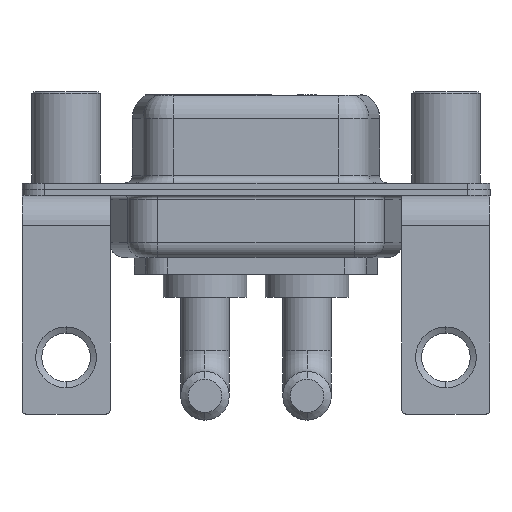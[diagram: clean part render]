
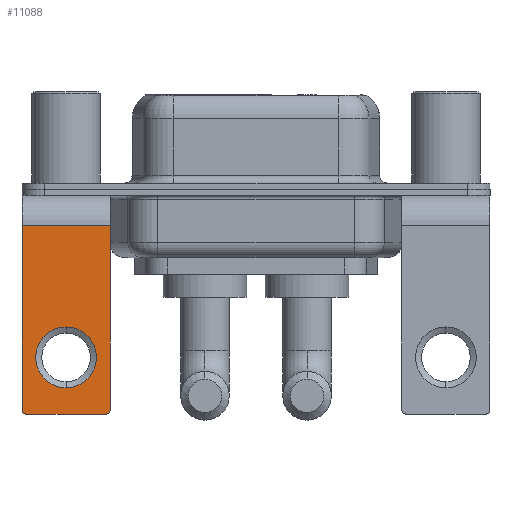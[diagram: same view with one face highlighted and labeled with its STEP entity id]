
A CAD part, front view. The second image highlights one B-rep face of the part: STEP entity #11088.
In plain terms, the highlighted planar face has unit normal (0, -1, 0).
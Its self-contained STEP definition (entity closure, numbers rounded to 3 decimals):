
#146 = LINE ( 'NONE', #1352, #6501 ) ;
#164 = ORIENTED_EDGE ( 'NONE', *, *, #9852, .F. ) ;
#209 = VECTOR ( 'NONE', #15672, 1000. ) ;
#387 = AXIS2_PLACEMENT_3D ( 'NONE', #13429, #12465, #3819 ) ;
#992 = VERTEX_POINT ( 'NONE', #1568 ) ;
#1039 = VERTEX_POINT ( 'NONE', #6690 ) ;
#1127 = VERTEX_POINT ( 'NONE', #11657 ) ;
#1352 = CARTESIAN_POINT ( 'NONE',  ( 2.9, -6.25, -14.8 ) ) ;
#1568 = CARTESIAN_POINT ( 'NONE',  ( 2.65, -6.25, -14.8 ) ) ;
#1747 = ORIENTED_EDGE ( 'NONE', *, *, #2289, .T. ) ;
#1815 = CIRCLE ( 'NONE', #6667, 0.25 ) ;
#2026 = CARTESIAN_POINT ( 'NONE',  ( 2.65, -6.25, -14.55 ) ) ;
#2289 = EDGE_CURVE ( 'NONE', #1127, #10317, #7300, .T. ) ;
#2880 = EDGE_CURVE ( 'NONE', #12796, #14570, #13454, .T. ) ;
#3440 = CIRCLE ( 'NONE', #14408, 0.25 ) ;
#3556 = VECTOR ( 'NONE', #14401, 1000. ) ;
#3585 = EDGE_LOOP ( 'NONE', ( #1747, #15638 ) ) ;
#3605 = CARTESIAN_POINT ( 'NONE',  ( 2.9, -6.25, -2.4 ) ) ;
#3757 = DIRECTION ( 'NONE',  ( 0., 0., 1. ) ) ;
#3819 = DIRECTION ( 'NONE',  ( 0., 0., 1. ) ) ;
#4032 = LINE ( 'NONE', #4910, #9857 ) ;
#4249 = DIRECTION ( 'NONE',  ( 0., 0., 1. ) ) ;
#4501 = CARTESIAN_POINT ( 'NONE',  ( 2.9, -6.25, -2.4 ) ) ;
#4638 = ORIENTED_EDGE ( 'NONE', *, *, #9647, .T. ) ;
#4791 = ORIENTED_EDGE ( 'NONE', *, *, #12128, .T. ) ;
#4910 = CARTESIAN_POINT ( 'NONE',  ( -2.9, -6.25, -2.4 ) ) ;
#4927 = EDGE_CURVE ( 'NONE', #10317, #1127, #7939, .T. ) ;
#4948 = EDGE_CURVE ( 'NONE', #992, #9258, #1815, .T. ) ;
#5245 = EDGE_LOOP ( 'NONE', ( #4791, #4638, #164, #15723, #7160, #8652 ) ) ;
#5376 = CARTESIAN_POINT ( 'NONE',  ( 0., -6.25, -11.07 ) ) ;
#6077 = PLANE ( 'NONE',  #9336 ) ;
#6238 = DIRECTION ( 'NONE',  ( -1., 0., 0. ) ) ;
#6501 = VECTOR ( 'NONE', #6238, 1000. ) ;
#6667 = AXIS2_PLACEMENT_3D ( 'NONE', #2026, #15224, #4249 ) ;
#6690 = CARTESIAN_POINT ( 'NONE',  ( -2.9, -6.25, -14.55 ) ) ;
#7160 = ORIENTED_EDGE ( 'NONE', *, *, #8058, .F. ) ;
#7300 = CIRCLE ( 'NONE', #387, 2. ) ;
#7939 = CIRCLE ( 'NONE', #9989, 2. ) ;
#8058 = EDGE_CURVE ( 'NONE', #12796, #9258, #9831, .T. ) ;
#8113 = DIRECTION ( 'NONE',  ( 0., 0., 1. ) ) ;
#8330 = CARTESIAN_POINT ( 'NONE',  ( -2.65, -6.25, -14.55 ) ) ;
#8478 = CARTESIAN_POINT ( 'NONE',  ( -2.9, -6.25, -2.4 ) ) ;
#8572 = DIRECTION ( 'NONE',  ( 0., 1., 0. ) ) ;
#8652 = ORIENTED_EDGE ( 'NONE', *, *, #2880, .T. ) ;
#8704 = CARTESIAN_POINT ( 'NONE',  ( -2.65, -6.25, -14.8 ) ) ;
#8922 = DIRECTION ( 'NONE',  ( 0., 0., -1. ) ) ;
#9253 = CARTESIAN_POINT ( 'NONE',  ( 0., -6.25, -9.07 ) ) ;
#9258 = VERTEX_POINT ( 'NONE', #15129 ) ;
#9336 = AXIS2_PLACEMENT_3D ( 'NONE', #4501, #8572, #3757 ) ;
#9647 = EDGE_CURVE ( 'NONE', #1039, #11623, #3440, .T. ) ;
#9831 = LINE ( 'NONE', #14714, #209 ) ;
#9852 = EDGE_CURVE ( 'NONE', #992, #11623, #146, .T. ) ;
#9857 = VECTOR ( 'NONE', #8922, 1000. ) ;
#9989 = AXIS2_PLACEMENT_3D ( 'NONE', #5376, #14183, #8113 ) ;
#10317 = VERTEX_POINT ( 'NONE', #9253 ) ;
#10674 = FACE_OUTER_BOUND ( 'NONE', #5245, .T. ) ;
#11088 = ADVANCED_FACE ( 'NONE', ( #15389, #10674 ), #6077, .F. ) ;
#11623 = VERTEX_POINT ( 'NONE', #8704 ) ;
#11657 = CARTESIAN_POINT ( 'NONE',  ( 0., -6.25, -13.07 ) ) ;
#12128 = EDGE_CURVE ( 'NONE', #14570, #1039, #4032, .T. ) ;
#12465 = DIRECTION ( 'NONE',  ( 0., 1., 0. ) ) ;
#12796 = VERTEX_POINT ( 'NONE', #13292 ) ;
#13208 = DIRECTION ( 'NONE',  ( 0., -1., 0. ) ) ;
#13292 = CARTESIAN_POINT ( 'NONE',  ( 2.9, -6.25, -2.4 ) ) ;
#13429 = CARTESIAN_POINT ( 'NONE',  ( 0., -6.25, -11.07 ) ) ;
#13454 = LINE ( 'NONE', #3605, #3556 ) ;
#14183 = DIRECTION ( 'NONE',  ( 0., 1., 0. ) ) ;
#14401 = DIRECTION ( 'NONE',  ( -1., 0., 0. ) ) ;
#14408 = AXIS2_PLACEMENT_3D ( 'NONE', #8330, #13208, #14552 ) ;
#14552 = DIRECTION ( 'NONE',  ( 0., 0., 1. ) ) ;
#14570 = VERTEX_POINT ( 'NONE', #8478 ) ;
#14714 = CARTESIAN_POINT ( 'NONE',  ( 2.9, -6.25, -2.4 ) ) ;
#15129 = CARTESIAN_POINT ( 'NONE',  ( 2.9, -6.25, -14.55 ) ) ;
#15224 = DIRECTION ( 'NONE',  ( 0., -1., 0. ) ) ;
#15389 = FACE_BOUND ( 'NONE', #3585, .T. ) ;
#15638 = ORIENTED_EDGE ( 'NONE', *, *, #4927, .T. ) ;
#15672 = DIRECTION ( 'NONE',  ( 0., 0., -1. ) ) ;
#15723 = ORIENTED_EDGE ( 'NONE', *, *, #4948, .T. ) ;
